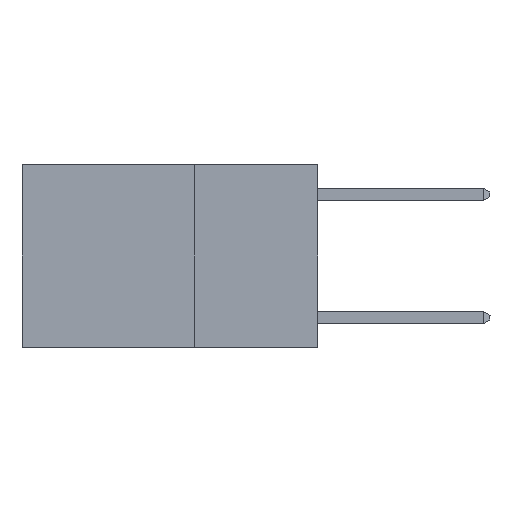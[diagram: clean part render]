
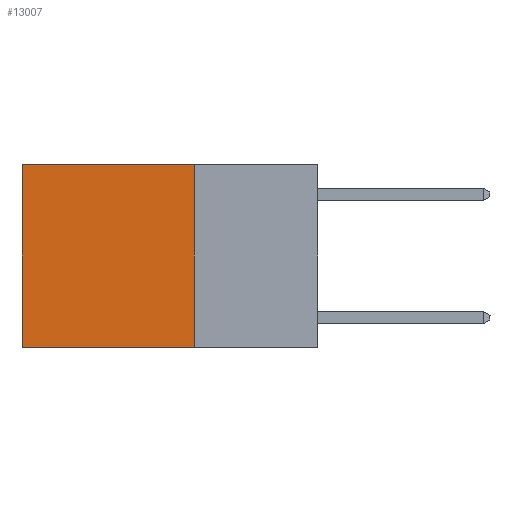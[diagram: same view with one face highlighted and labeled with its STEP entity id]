
A CAD part, left-side view. The second image highlights one B-rep face of the part: STEP entity #13007.
In plain terms, the highlighted planar face has unit normal (-1, 0, 0).
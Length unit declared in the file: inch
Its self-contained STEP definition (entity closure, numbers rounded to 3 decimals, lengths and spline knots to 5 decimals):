
#549 = CARTESIAN_POINT ( 'NONE',  ( 0.2625, 0.25, 0. ) ) ;
#796 = ORIENTED_EDGE ( 'NONE', *, *, #13083, .T. ) ;
#1025 = VECTOR ( 'NONE', #6983, 39.37008 ) ;
#1192 = VERTEX_POINT ( 'NONE', #11800 ) ;
#1670 = PLANE ( 'NONE',  #10898 ) ;
#1915 = EDGE_CURVE ( 'NONE', #13262, #2747, #7643, .T. ) ;
#2696 = CARTESIAN_POINT ( 'NONE',  ( 0.2625, 0.6, 0. ) ) ;
#2715 = ORIENTED_EDGE ( 'NONE', *, *, #14940, .F. ) ;
#2747 = VERTEX_POINT ( 'NONE', #7661 ) ;
#2817 = CARTESIAN_POINT ( 'NONE',  ( 0.2625, 0.6, -0.37 ) ) ;
#3949 = EDGE_CURVE ( 'NONE', #1192, #7526, #4996, .T. ) ;
#4996 = LINE ( 'NONE', #2696, #9411 ) ;
#5113 = ORIENTED_EDGE ( 'NONE', *, *, #3949, .T. ) ;
#5354 = CARTESIAN_POINT ( 'NONE',  ( 0.2625, 0.25, 0. ) ) ;
#6740 = FACE_OUTER_BOUND ( 'NONE', #14201, .T. ) ;
#6889 = CARTESIAN_POINT ( 'NONE',  ( 0.2625, 0.25, 0. ) ) ;
#6983 = DIRECTION ( 'NONE',  ( 0., 1., 0. ) ) ;
#7526 = VERTEX_POINT ( 'NONE', #2817 ) ;
#7643 = LINE ( 'NONE', #549, #9274 ) ;
#7661 = CARTESIAN_POINT ( 'NONE',  ( 0.2625, 0.25, -0.37 ) ) ;
#8113 = VECTOR ( 'NONE', #10710, 39.37008 ) ;
#9274 = VECTOR ( 'NONE', #12135, 39.37008 ) ;
#9411 = VECTOR ( 'NONE', #11754, 39.37008 ) ;
#10710 = DIRECTION ( 'NONE',  ( 0., 1., 0. ) ) ;
#10898 = AXIS2_PLACEMENT_3D ( 'NONE', #6889, #13149, #15857 ) ;
#11070 = CARTESIAN_POINT ( 'NONE',  ( 0.2625, 0.25, 0. ) ) ;
#11754 = DIRECTION ( 'NONE',  ( 0., 0., -1. ) ) ;
#11800 = CARTESIAN_POINT ( 'NONE',  ( 0.2625, 0.6, 0. ) ) ;
#11884 = ORIENTED_EDGE ( 'NONE', *, *, #1915, .F. ) ;
#12135 = DIRECTION ( 'NONE',  ( 0., 0., -1. ) ) ;
#13007 = ADVANCED_FACE ( 'NONE', ( #6740 ), #1670, .F. ) ;
#13083 = EDGE_CURVE ( 'NONE', #13262, #1192, #14831, .T. ) ;
#13149 = DIRECTION ( 'NONE',  ( 1., 0., 0. ) ) ;
#13262 = VERTEX_POINT ( 'NONE', #11070 ) ;
#14121 = LINE ( 'NONE', #14688, #1025 ) ;
#14201 = EDGE_LOOP ( 'NONE', ( #5113, #2715, #11884, #796 ) ) ;
#14688 = CARTESIAN_POINT ( 'NONE',  ( 0.2625, 0.25, -0.37 ) ) ;
#14831 = LINE ( 'NONE', #5354, #8113 ) ;
#14940 = EDGE_CURVE ( 'NONE', #2747, #7526, #14121, .T. ) ;
#15857 = DIRECTION ( 'NONE',  ( 0., 0., -1. ) ) ;
